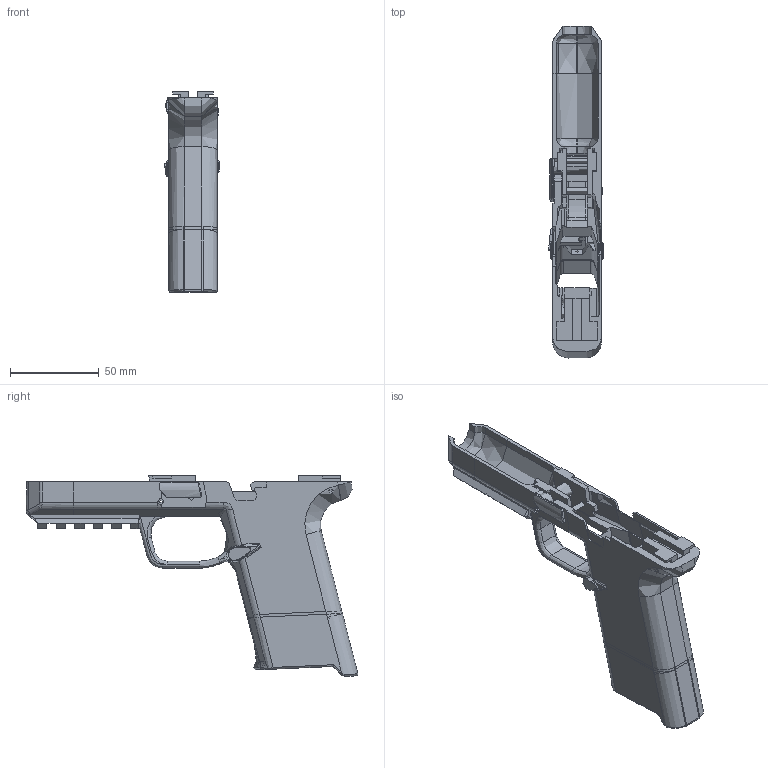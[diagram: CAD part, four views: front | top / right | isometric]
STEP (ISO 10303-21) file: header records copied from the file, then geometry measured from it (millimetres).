
FILE_DESCRIPTION(/* description */ (''),/* implementation_level */ '2;1');
FILE_NAME(/* name */ 'M&P 9 Assembly + Picatinny - Full Size Slide M2.0.step',/* time_stamp */ '2022-02-23T00:58:53-05:00',/* author */ (''),/* organization */ (''),/* preprocessor_version */ 'ST-DEVELOPER v18.1',/* originating_system */ 'Autodesk Translation Framework v10.13.0.1454',/* authorisation */ '');
FILE_SCHEMA (('AUTOMOTIVE_DESIGN { 1 0 10303 214 3 1 1 }'));
Length unit declared in the file: millimetre
Products named in the file (13): M&P 9 M2.0 Standard Length Slide - Picatinny; M&P 9 Reference v116; Rear Fire Control Group Pin; Front Locking Block Group Pin; Trigger Pin; Locking Block; Disassembly Lug; Rear Fire Control Group; Frame; Trigger Guard and Magwell; Fitment Section; Full-Size Magwell Body; Magazine Release Button
Assembly tree (12 placements, depth 4):
  M&P 9 M2.0 Standard Length Slide - Picatinny
    M&P 9 Reference v116
      Rear Fire Control Group Pin
      Front Locking Block Group Pin
      Trigger Pin
      Locking Block
      Disassembly Lug
      Rear Fire Control Group
      Frame
        Trigger Guard and Magwell
        Fitment Section
        Full-Size Magwell Body
      Magazine Release Button
Bounding box: 30.95 x 186.75 x 113.13 mm (x, y, z)
Volume: 110080.5 mm3; surface area: 61585.7 mm2
Topology: 13 solids, 13 shells, 749 faces, 2031 edges, 1292 vertices
Faces by surface type: plane 398, cylinder 209, bspline 115, torus 21, sphere 4, cone 2
Full cylindrical faces by diameter (mm): 1.35 x2, 1.5 x3, 3.15 x2, 3.18 x3, 3.2 x2, 3.361 x2, 3.5 x1, 3.55 x4, 4.7 x1, 5.1 x1, 6.3 x1, 7.7 x1, 8.8 x1, 9 x2
Entity records: 27762 total; most frequent: CARTESIAN_POINT 8868, ORIENTED_EDGE 4040, DIRECTION 3657, EDGE_CURVE 2020, VERTEX_POINT 1292, LINE 1249, VECTOR 1249, AXIS2_PLACEMENT_3D 1204
